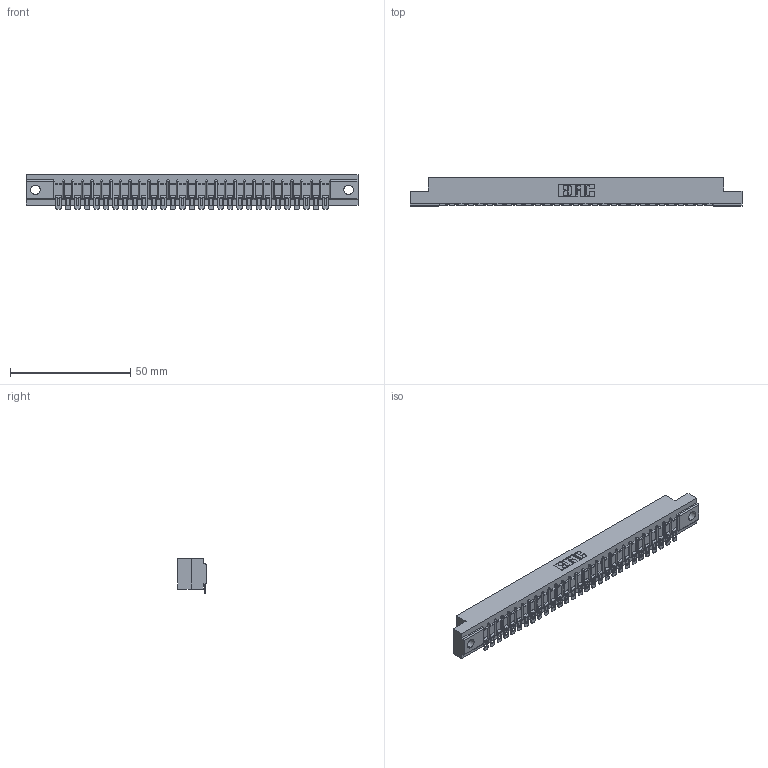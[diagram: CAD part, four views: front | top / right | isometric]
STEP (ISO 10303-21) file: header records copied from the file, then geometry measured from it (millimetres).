
FILE_DESCRIPTION (( 'STEP AP203' ), '1' );
FILE_NAME ('307-029-454-102.STEP', '2020-09-28T09:58:30', ( '' ), ( '' ), 'SwSTEP 2.0', 'SolidWorks 2020', '' );
FILE_SCHEMA (( 'CONFIG_CONTROL_DESIGN' ));
Length unit declared in the file: inch
Products named in the file (3): 307 Part_.128 Dia Mounting Holes; 307-029-454-102; 307-290-002_554
Assembly tree (30 placements, depth 2):
  307-029-454-102
    307 Part_.128 Dia Mounting Holes
    307-290-002_554  x29
Bounding box: 137.92 x 12.01 x 14.52 mm (x, y, z)
Volume: 14585.1 mm3; surface area: 17969.2 mm2
Topology: 30 solids, 30 shells, 2497 faces, 7660 edges, 5024 vertices
Faces by surface type: plane 1404, cylinder 1033, sphere 60
Entity records: 27431 total; most frequent: CARTESIAN_POINT 4626, ORIENTED_EDGE 4616, DIRECTION 4506, EDGE_CURVE 2308, VECTOR 1754, LINE 1754, VERTEX_POINT 1496, AXIS2_PLACEMENT_3D 1376
